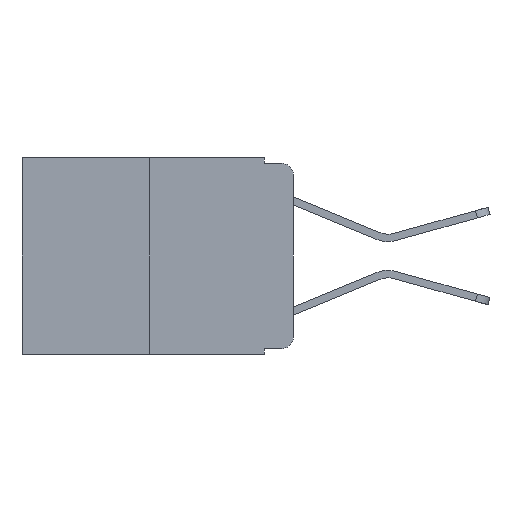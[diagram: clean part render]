
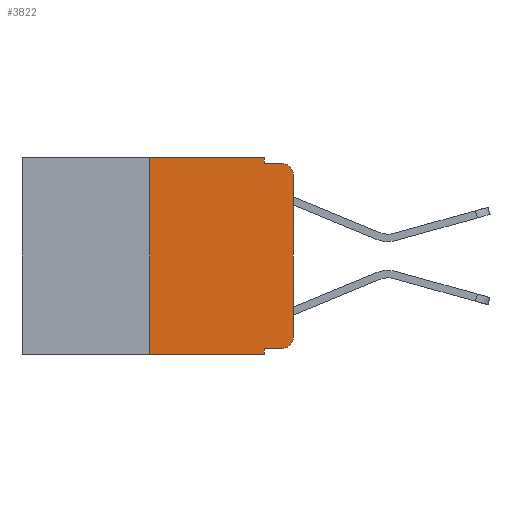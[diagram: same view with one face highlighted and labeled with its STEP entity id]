
A CAD part, left-side view. The second image highlights one B-rep face of the part: STEP entity #3822.
In plain terms, the highlighted planar face has unit normal (-1, 0, 0).
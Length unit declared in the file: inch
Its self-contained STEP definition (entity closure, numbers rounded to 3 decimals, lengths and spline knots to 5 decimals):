
#10 = DIRECTION ( 'NONE',  ( -1., 0., 0. ) ) ;
#131 = VECTOR ( 'NONE', #6864, 39.37008 ) ;
#296 = LINE ( 'NONE', #1048, #6176 ) ;
#306 = CARTESIAN_POINT ( 'NONE',  ( 0., 0.473, 0. ) ) ;
#310 = LINE ( 'NONE', #6737, #6192 ) ;
#460 = VERTEX_POINT ( 'NONE', #5371 ) ;
#511 = VERTEX_POINT ( 'NONE', #2947 ) ;
#572 = CARTESIAN_POINT ( 'NONE',  ( 0., 0.02, -0.01 ) ) ;
#622 = CARTESIAN_POINT ( 'NONE',  ( 0., 0.051, -0.01 ) ) ;
#990 = VERTEX_POINT ( 'NONE', #8444 ) ;
#1048 = CARTESIAN_POINT ( 'NONE',  ( 0., 0., 0. ) ) ;
#1215 = VERTEX_POINT ( 'NONE', #622 ) ;
#1229 = AXIS2_PLACEMENT_3D ( 'NONE', #2661, #7686, #3416 ) ;
#1331 = VECTOR ( 'NONE', #9393, 39.37008 ) ;
#1455 = VECTOR ( 'NONE', #2085, 39.37008 ) ;
#1701 = CIRCLE ( 'NONE', #4759, 0.02 ) ;
#1874 = EDGE_CURVE ( 'NONE', #6891, #511, #5339, .T. ) ;
#2085 = DIRECTION ( 'NONE',  ( 0., -1., 0. ) ) ;
#2517 = CARTESIAN_POINT ( 'NONE',  ( 0., 0., -0.313 ) ) ;
#2574 = VERTEX_POINT ( 'NONE', #4865 ) ;
#2661 = CARTESIAN_POINT ( 'NONE',  ( 0., 0.02, -0.03 ) ) ;
#2884 = VECTOR ( 'NONE', #4743, 39.37008 ) ;
#2947 = CARTESIAN_POINT ( 'NONE',  ( 0., 0.25, 0. ) ) ;
#3291 = ORIENTED_EDGE ( 'NONE', *, *, #8800, .F. ) ;
#3305 = EDGE_CURVE ( 'NONE', #6765, #2574, #296, .T. ) ;
#3353 = VECTOR ( 'NONE', #7071, 39.37008 ) ;
#3406 = ORIENTED_EDGE ( 'NONE', *, *, #7830, .T. ) ;
#3416 = DIRECTION ( 'NONE',  ( 0., 0., -1. ) ) ;
#3425 = EDGE_CURVE ( 'NONE', #6103, #1215, #7160, .T. ) ;
#3635 = DIRECTION ( 'NONE',  ( 0., 0., -1. ) ) ;
#3822 = ADVANCED_FACE ( 'NONE', ( #8968 ), #8458, .F. ) ;
#3973 = EDGE_LOOP ( 'NONE', ( #8380, #3406, #8823, #8693, #8700, #5174, #8701, #3291, #4570, #9010 ) ) ;
#4054 = CARTESIAN_POINT ( 'NONE',  ( 0., 0.051, -0.333 ) ) ;
#4334 = LINE ( 'NONE', #5405, #131 ) ;
#4382 = EDGE_CURVE ( 'NONE', #1215, #4787, #4334, .T. ) ;
#4570 = ORIENTED_EDGE ( 'NONE', *, *, #8341, .T. ) ;
#4681 = EDGE_CURVE ( 'NONE', #6891, #990, #7349, .T. ) ;
#4697 = CARTESIAN_POINT ( 'NONE',  ( 0., 0.02, -0.313 ) ) ;
#4743 = DIRECTION ( 'NONE',  ( 0., -1., 0. ) ) ;
#4759 = AXIS2_PLACEMENT_3D ( 'NONE', #4697, #10, #5418 ) ;
#4787 = VERTEX_POINT ( 'NONE', #572 ) ;
#4865 = CARTESIAN_POINT ( 'NONE',  ( 0., 0., -0.03 ) ) ;
#5174 = ORIENTED_EDGE ( 'NONE', *, *, #1874, .F. ) ;
#5339 = LINE ( 'NONE', #8970, #1331 ) ;
#5371 = CARTESIAN_POINT ( 'NONE',  ( 0., 0.02, -0.333 ) ) ;
#5405 = CARTESIAN_POINT ( 'NONE',  ( 0., 0.051, -0.01 ) ) ;
#5418 = DIRECTION ( 'NONE',  ( 0., 0., -1. ) ) ;
#5525 = EDGE_CURVE ( 'NONE', #460, #6765, #1701, .T. ) ;
#5690 = DIRECTION ( 'NONE',  ( 0., -1., 0. ) ) ;
#5889 = CARTESIAN_POINT ( 'NONE',  ( 0., 0.25, -0.343 ) ) ;
#6089 = CARTESIAN_POINT ( 'NONE',  ( 0., 0.051, 0. ) ) ;
#6103 = VERTEX_POINT ( 'NONE', #6089 ) ;
#6176 = VECTOR ( 'NONE', #8423, 39.37008 ) ;
#6192 = VECTOR ( 'NONE', #7443, 39.37008 ) ;
#6402 = LINE ( 'NONE', #306, #8244 ) ;
#6725 = VERTEX_POINT ( 'NONE', #6802 ) ;
#6737 = CARTESIAN_POINT ( 'NONE',  ( 0., 0.051, 0. ) ) ;
#6765 = VERTEX_POINT ( 'NONE', #2517 ) ;
#6802 = CARTESIAN_POINT ( 'NONE',  ( 0., 0.051, -0.333 ) ) ;
#6864 = DIRECTION ( 'NONE',  ( 0., -1., 0. ) ) ;
#6891 = VERTEX_POINT ( 'NONE', #5889 ) ;
#7071 = DIRECTION ( 'NONE',  ( 0., 0., -1. ) ) ;
#7160 = LINE ( 'NONE', #8686, #3353 ) ;
#7194 = CARTESIAN_POINT ( 'NONE',  ( 0., 0.473, -0.343 ) ) ;
#7326 = EDGE_CURVE ( 'NONE', #511, #6103, #6402, .T. ) ;
#7349 = LINE ( 'NONE', #7194, #1455 ) ;
#7443 = DIRECTION ( 'NONE',  ( 0., 0., -1. ) ) ;
#7686 = DIRECTION ( 'NONE',  ( -1., 0., 0. ) ) ;
#7830 = EDGE_CURVE ( 'NONE', #2574, #4787, #9196, .T. ) ;
#8244 = VECTOR ( 'NONE', #5690, 39.37008 ) ;
#8341 = EDGE_CURVE ( 'NONE', #6725, #460, #8764, .T. ) ;
#8380 = ORIENTED_EDGE ( 'NONE', *, *, #3305, .T. ) ;
#8423 = DIRECTION ( 'NONE',  ( 0., 0., 1. ) ) ;
#8444 = CARTESIAN_POINT ( 'NONE',  ( 0., 0.051, -0.343 ) ) ;
#8458 = PLANE ( 'NONE',  #9085 ) ;
#8513 = CARTESIAN_POINT ( 'NONE',  ( 0., 0.473, 0. ) ) ;
#8686 = CARTESIAN_POINT ( 'NONE',  ( 0., 0.051, 0. ) ) ;
#8693 = ORIENTED_EDGE ( 'NONE', *, *, #3425, .F. ) ;
#8700 = ORIENTED_EDGE ( 'NONE', *, *, #7326, .F. ) ;
#8701 = ORIENTED_EDGE ( 'NONE', *, *, #4681, .T. ) ;
#8764 = LINE ( 'NONE', #4054, #2884 ) ;
#8800 = EDGE_CURVE ( 'NONE', #6725, #990, #310, .T. ) ;
#8823 = ORIENTED_EDGE ( 'NONE', *, *, #4382, .F. ) ;
#8957 = DIRECTION ( 'NONE',  ( 1., 0., 0. ) ) ;
#8968 = FACE_OUTER_BOUND ( 'NONE', #3973, .T. ) ;
#8970 = CARTESIAN_POINT ( 'NONE',  ( 0., 0.25, 0. ) ) ;
#9010 = ORIENTED_EDGE ( 'NONE', *, *, #5525, .T. ) ;
#9085 = AXIS2_PLACEMENT_3D ( 'NONE', #8513, #8957, #3635 ) ;
#9196 = CIRCLE ( 'NONE', #1229, 0.02 ) ;
#9393 = DIRECTION ( 'NONE',  ( 0., 0., 1. ) ) ;
